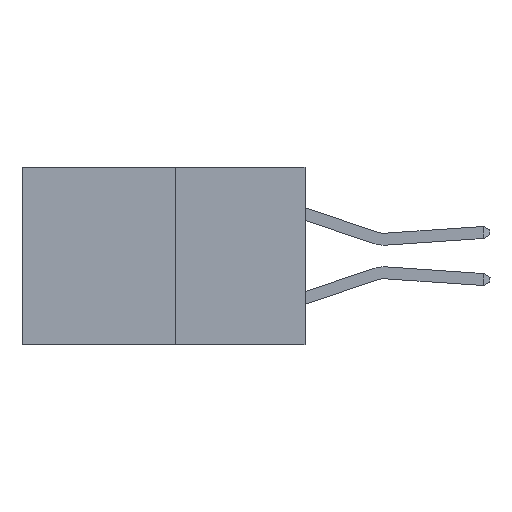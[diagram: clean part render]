
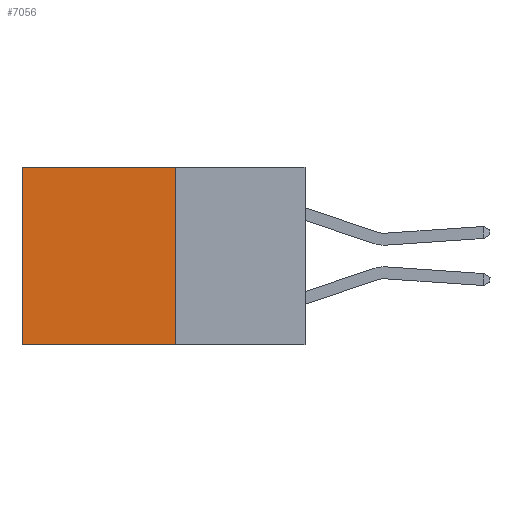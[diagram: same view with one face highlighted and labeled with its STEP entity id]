
A CAD part, left-side view. The second image highlights one B-rep face of the part: STEP entity #7056.
In plain terms, the highlighted planar face has unit normal (-1, 0, 0).
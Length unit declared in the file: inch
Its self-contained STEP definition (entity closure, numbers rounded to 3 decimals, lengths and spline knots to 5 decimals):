
#492 = DIRECTION ( 'NONE',  ( 0., 1., 0. ) ) ;
#759 = ORIENTED_EDGE ( 'NONE', *, *, #15093, .T. ) ;
#1081 = DIRECTION ( 'NONE',  ( 0., 0., -1. ) ) ;
#2291 = VECTOR ( 'NONE', #492, 39.37008 ) ;
#2358 = CARTESIAN_POINT ( 'NONE',  ( 0.277, 0.27, -0.37 ) ) ;
#3088 = EDGE_LOOP ( 'NONE', ( #17901, #15099, #15986, #759 ) ) ;
#3192 = CARTESIAN_POINT ( 'NONE',  ( 0.277, 0.59, -0.37 ) ) ;
#3520 = DIRECTION ( 'NONE',  ( 0., 0., -1. ) ) ;
#4045 = EDGE_CURVE ( 'NONE', #17137, #16088, #9990, .T. ) ;
#4376 = LINE ( 'NONE', #18555, #15480 ) ;
#4940 = CARTESIAN_POINT ( 'NONE',  ( 0.277, 0.27, 0. ) ) ;
#4991 = VERTEX_POINT ( 'NONE', #12326 ) ;
#5016 = VECTOR ( 'NONE', #3520, 39.37008 ) ;
#5933 = CARTESIAN_POINT ( 'NONE',  ( 0.277, 0.27, -0.37 ) ) ;
#5994 = DIRECTION ( 'NONE',  ( 0., 0., -1. ) ) ;
#6273 = DIRECTION ( 'NONE',  ( 0., 1., 0. ) ) ;
#6381 = AXIS2_PLACEMENT_3D ( 'NONE', #6675, #6517, #5994 ) ;
#6517 = DIRECTION ( 'NONE',  ( 1., 0., 0. ) ) ;
#6675 = CARTESIAN_POINT ( 'NONE',  ( 0.277, 0.27, -0.37 ) ) ;
#7056 = ADVANCED_FACE ( 'NONE', ( #8243 ), #7880, .F. ) ;
#7880 = PLANE ( 'NONE',  #6381 ) ;
#8243 = FACE_OUTER_BOUND ( 'NONE', #3088, .T. ) ;
#9238 = LINE ( 'NONE', #10669, #5016 ) ;
#9539 = VECTOR ( 'NONE', #6273, 39.37008 ) ;
#9990 = LINE ( 'NONE', #5933, #9539 ) ;
#10001 = VERTEX_POINT ( 'NONE', #4940 ) ;
#10099 = LINE ( 'NONE', #18008, #2291 ) ;
#10669 = CARTESIAN_POINT ( 'NONE',  ( 0.277, 0.27, -0.37 ) ) ;
#10721 = EDGE_CURVE ( 'NONE', #10001, #17137, #9238, .T. ) ;
#12326 = CARTESIAN_POINT ( 'NONE',  ( 0.277, 0.59, 0. ) ) ;
#13353 = EDGE_CURVE ( 'NONE', #4991, #16088, #4376, .T. ) ;
#15093 = EDGE_CURVE ( 'NONE', #10001, #4991, #10099, .T. ) ;
#15099 = ORIENTED_EDGE ( 'NONE', *, *, #4045, .F. ) ;
#15480 = VECTOR ( 'NONE', #1081, 39.37008 ) ;
#15986 = ORIENTED_EDGE ( 'NONE', *, *, #10721, .F. ) ;
#16088 = VERTEX_POINT ( 'NONE', #3192 ) ;
#17137 = VERTEX_POINT ( 'NONE', #2358 ) ;
#17901 = ORIENTED_EDGE ( 'NONE', *, *, #13353, .T. ) ;
#18008 = CARTESIAN_POINT ( 'NONE',  ( 0.277, 0.27, 0. ) ) ;
#18555 = CARTESIAN_POINT ( 'NONE',  ( 0.277, 0.59, -0.37 ) ) ;
